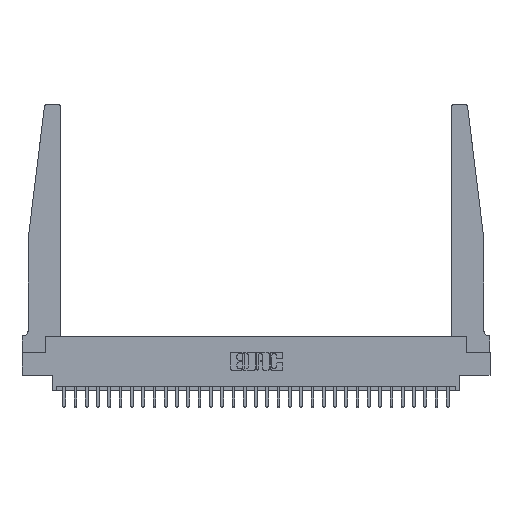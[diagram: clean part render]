
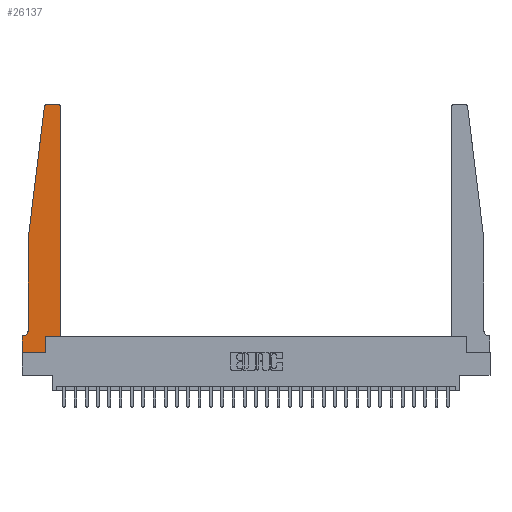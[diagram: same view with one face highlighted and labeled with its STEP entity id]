
A CAD part, top view. The second image highlights one B-rep face of the part: STEP entity #26137.
In plain terms, the highlighted planar face has unit normal (0, 0, 1).
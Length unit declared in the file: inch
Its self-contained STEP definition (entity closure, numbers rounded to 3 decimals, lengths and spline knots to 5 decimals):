
#29 = EDGE_CURVE ( 'NONE', #204, #25537, #5910, .T. ) ;
#198 = VERTEX_POINT ( 'NONE', #672 ) ;
#204 = VERTEX_POINT ( 'NONE', #4702 ) ;
#672 = CARTESIAN_POINT ( 'NONE',  ( 0.425, 0.18, 0.37 ) ) ;
#723 = EDGE_CURVE ( 'NONE', #15489, #204, #4778, .T. ) ;
#749 = VERTEX_POINT ( 'NONE', #11736 ) ;
#931 = PLANE ( 'NONE',  #4134 ) ;
#1118 = ORIENTED_EDGE ( 'NONE', *, *, #5520, .T. ) ;
#1181 = ORIENTED_EDGE ( 'NONE', *, *, #20159, .T. ) ;
#1259 = LINE ( 'NONE', #10296, #27841 ) ;
#1281 = CARTESIAN_POINT ( 'NONE',  ( 0.2605, 0.18, 0.37 ) ) ;
#1773 = CARTESIAN_POINT ( 'NONE',  ( 0.065, 1.25, 0.37 ) ) ;
#1979 = EDGE_CURVE ( 'NONE', #198, #749, #4522, .T. ) ;
#2194 = DIRECTION ( 'NONE',  ( 0., 0., 1. ) ) ;
#2202 = CARTESIAN_POINT ( 'NONE',  ( 0.25, 2.75, 0.37 ) ) ;
#2413 = DIRECTION ( 'NONE',  ( 0., -1., 0. ) ) ;
#2672 = VECTOR ( 'NONE', #8713, 39.37008 ) ;
#2714 = ORIENTED_EDGE ( 'NONE', *, *, #19194, .T. ) ;
#2971 = CARTESIAN_POINT ( 'NONE',  ( 0., 0.1875, 0.37 ) ) ;
#4066 = CIRCLE ( 'NONE', #22947, 0.03 ) ;
#4134 = AXIS2_PLACEMENT_3D ( 'NONE', #8434, #6206, #5366 ) ;
#4522 = LINE ( 'NONE', #24824, #10568 ) ;
#4702 = CARTESIAN_POINT ( 'NONE',  ( 0., 0., 0.37 ) ) ;
#4778 = LINE ( 'NONE', #13655, #24641 ) ;
#4956 = VERTEX_POINT ( 'NONE', #5189 ) ;
#5189 = CARTESIAN_POINT ( 'NONE',  ( 0.015, 0.1875, 0.37 ) ) ;
#5366 = DIRECTION ( 'NONE',  ( 1., 0., 0. ) ) ;
#5520 = EDGE_CURVE ( 'NONE', #749, #25956, #4066, .T. ) ;
#5910 = LINE ( 'NONE', #13160, #14257 ) ;
#6076 = CARTESIAN_POINT ( 'NONE',  ( 0.24675, 2.72367, 0.37 ) ) ;
#6206 = DIRECTION ( 'NONE',  ( 0., 0., 1. ) ) ;
#6209 = ORIENTED_EDGE ( 'NONE', *, *, #1979, .T. ) ;
#6369 = ORIENTED_EDGE ( 'NONE', *, *, #27138, .T. ) ;
#6445 = ORIENTED_EDGE ( 'NONE', *, *, #24920, .T. ) ;
#6654 = CARTESIAN_POINT ( 'NONE',  ( 0.065, 0.2375, 0.37 ) ) ;
#6678 = AXIS2_PLACEMENT_3D ( 'NONE', #19772, #21689, #12952 ) ;
#7903 = VERTEX_POINT ( 'NONE', #1281 ) ;
#8175 = VECTOR ( 'NONE', #12656, 39.37008 ) ;
#8290 = DIRECTION ( 'NONE',  ( 1., 0., 0. ) ) ;
#8434 = CARTESIAN_POINT ( 'NONE',  ( 0., 0.1875, 0.37 ) ) ;
#8713 = DIRECTION ( 'NONE',  ( 0., -1., 0. ) ) ;
#8718 = DIRECTION ( 'NONE',  ( 1., 0., 0. ) ) ;
#8865 = ORIENTED_EDGE ( 'NONE', *, *, #723, .T. ) ;
#8903 = VERTEX_POINT ( 'NONE', #6654 ) ;
#9008 = CARTESIAN_POINT ( 'NONE',  ( 0.27653, 2.72, 0.37 ) ) ;
#10296 = CARTESIAN_POINT ( 'NONE',  ( 0.065, 1.25, 0.37 ) ) ;
#10568 = VECTOR ( 'NONE', #25274, 39.37008 ) ;
#10764 = VERTEX_POINT ( 'NONE', #20962 ) ;
#10899 = CARTESIAN_POINT ( 'NONE',  ( 0.2605, 0., 0.37 ) ) ;
#11007 = CARTESIAN_POINT ( 'NONE',  ( 0.425, 0.18, 0.37 ) ) ;
#11736 = CARTESIAN_POINT ( 'NONE',  ( 0.425, 2.72, 0.37 ) ) ;
#12564 = AXIS2_PLACEMENT_3D ( 'NONE', #9008, #2194, #8718 ) ;
#12612 = EDGE_CURVE ( 'NONE', #4956, #15489, #23521, .T. ) ;
#12656 = DIRECTION ( 'NONE',  ( 1., 0., 0. ) ) ;
#12952 = DIRECTION ( 'NONE',  ( -1., 0., 0. ) ) ;
#13008 = EDGE_CURVE ( 'NONE', #10764, #15610, #13054, .T. ) ;
#13054 = CIRCLE ( 'NONE', #12564, 0.03 ) ;
#13091 = DIRECTION ( 'NONE',  ( 1., 0., 0. ) ) ;
#13160 = CARTESIAN_POINT ( 'NONE',  ( 0., 0., 0.37 ) ) ;
#13434 = VECTOR ( 'NONE', #13899, 39.37008 ) ;
#13655 = CARTESIAN_POINT ( 'NONE',  ( 0., 0., 0.37 ) ) ;
#13899 = DIRECTION ( 'NONE',  ( -1., 0., 0. ) ) ;
#14086 = CARTESIAN_POINT ( 'NONE',  ( 0.395, 2.75, 0.37 ) ) ;
#14257 = VECTOR ( 'NONE', #8290, 39.37008 ) ;
#15431 = VECTOR ( 'NONE', #23213, 39.37008 ) ;
#15489 = VERTEX_POINT ( 'NONE', #2971 ) ;
#15610 = VERTEX_POINT ( 'NONE', #6076 ) ;
#16694 = ORIENTED_EDGE ( 'NONE', *, *, #13008, .T. ) ;
#16758 = FACE_OUTER_BOUND ( 'NONE', #19205, .T. ) ;
#16843 = ORIENTED_EDGE ( 'NONE', *, *, #25155, .T. ) ;
#17525 = CARTESIAN_POINT ( 'NONE',  ( 0.395, 2.72, 0.37 ) ) ;
#17894 = DIRECTION ( 'NONE',  ( -1., 0., 0. ) ) ;
#18414 = ORIENTED_EDGE ( 'NONE', *, *, #29, .T. ) ;
#18496 = CARTESIAN_POINT ( 'NONE',  ( 0.065, 0.1875, 0.37 ) ) ;
#18638 = LINE ( 'NONE', #27693, #15431 ) ;
#18883 = EDGE_CURVE ( 'NONE', #8903, #4956, #19463, .T. ) ;
#19194 = EDGE_CURVE ( 'NONE', #7903, #198, #23898, .T. ) ;
#19205 = EDGE_LOOP ( 'NONE', ( #1181, #16694, #6369, #16843, #22516, #24373, #8865, #18414, #6445, #2714, #6209, #1118 ) ) ;
#19325 = DIRECTION ( 'NONE',  ( -0.122, -0.992, 0. ) ) ;
#19463 = CIRCLE ( 'NONE', #6678, 0.05 ) ;
#19772 = CARTESIAN_POINT ( 'NONE',  ( 0.015, 0.2375, 0.37 ) ) ;
#20159 = EDGE_CURVE ( 'NONE', #25956, #10764, #22186, .T. ) ;
#20470 = VERTEX_POINT ( 'NONE', #26052 ) ;
#20962 = CARTESIAN_POINT ( 'NONE',  ( 0.27653, 2.75, 0.37 ) ) ;
#21689 = DIRECTION ( 'NONE',  ( 0., 0., -1. ) ) ;
#22186 = LINE ( 'NONE', #2202, #28228 ) ;
#22516 = ORIENTED_EDGE ( 'NONE', *, *, #18883, .T. ) ;
#22947 = AXIS2_PLACEMENT_3D ( 'NONE', #17525, #23892, #13091 ) ;
#23213 = DIRECTION ( 'NONE',  ( 0., 1., 0. ) ) ;
#23521 = LINE ( 'NONE', #18496, #13434 ) ;
#23892 = DIRECTION ( 'NONE',  ( 0., 0., 1. ) ) ;
#23898 = LINE ( 'NONE', #11007, #8175 ) ;
#24373 = ORIENTED_EDGE ( 'NONE', *, *, #12612, .T. ) ;
#24641 = VECTOR ( 'NONE', #2413, 39.37008 ) ;
#24824 = CARTESIAN_POINT ( 'NONE',  ( 0.425, 0.18, 0.37 ) ) ;
#24920 = EDGE_CURVE ( 'NONE', #25537, #7903, #18638, .T. ) ;
#25155 = EDGE_CURVE ( 'NONE', #20470, #8903, #27083, .T. ) ;
#25274 = DIRECTION ( 'NONE',  ( 0., 1., 0. ) ) ;
#25537 = VERTEX_POINT ( 'NONE', #10899 ) ;
#25956 = VERTEX_POINT ( 'NONE', #14086 ) ;
#26052 = CARTESIAN_POINT ( 'NONE',  ( 0.065, 1.25, 0.37 ) ) ;
#26137 = ADVANCED_FACE ( 'NONE', ( #16758 ), #931, .T. ) ;
#27083 = LINE ( 'NONE', #1773, #2672 ) ;
#27138 = EDGE_CURVE ( 'NONE', #15610, #20470, #1259, .T. ) ;
#27693 = CARTESIAN_POINT ( 'NONE',  ( 0.2605, 0.18, 0.37 ) ) ;
#27841 = VECTOR ( 'NONE', #19325, 39.37008 ) ;
#28228 = VECTOR ( 'NONE', #17894, 39.37008 ) ;
